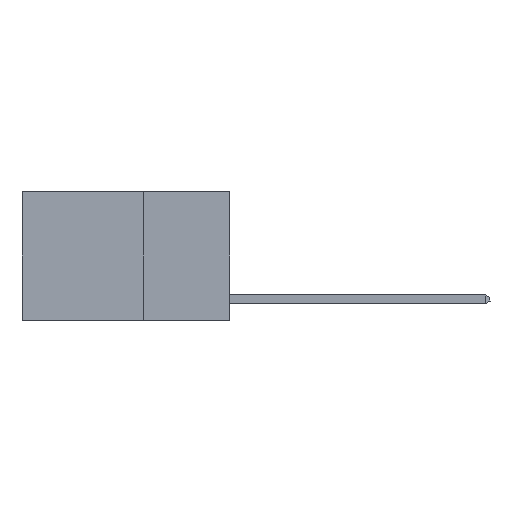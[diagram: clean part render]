
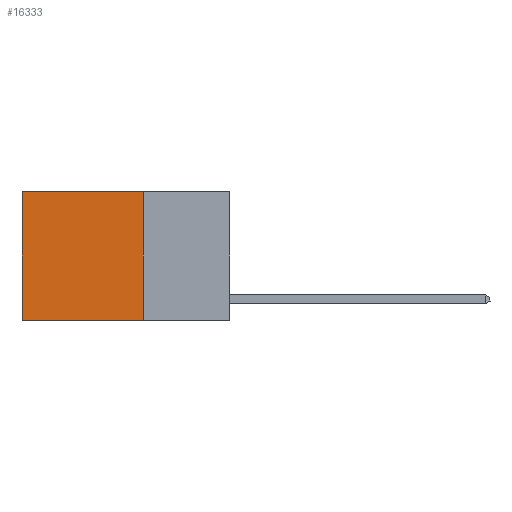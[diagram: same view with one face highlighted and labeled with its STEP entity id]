
A CAD part, left-side view. The second image highlights one B-rep face of the part: STEP entity #16333.
In plain terms, the highlighted planar face has unit normal (-1, 0, 0).
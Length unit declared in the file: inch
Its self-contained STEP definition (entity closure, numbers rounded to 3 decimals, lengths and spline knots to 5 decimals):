
#13 = EDGE_CURVE ( 'NONE', #12201, #6996, #4088, .T. ) ;
#409 = AXIS2_PLACEMENT_3D ( 'NONE', #1195, #7723, #7831 ) ;
#602 = VECTOR ( 'NONE', #15151, 39.37008 ) ;
#702 = CARTESIAN_POINT ( 'NONE',  ( 0.2625, 0.25, 0. ) ) ;
#754 = CARTESIAN_POINT ( 'NONE',  ( 0.2625, 0.25, -0.37 ) ) ;
#1195 = CARTESIAN_POINT ( 'NONE',  ( 0.2625, 0.25, 0. ) ) ;
#2214 = EDGE_CURVE ( 'NONE', #6996, #4383, #11823, .T. ) ;
#2834 = EDGE_LOOP ( 'NONE', ( #11402, #3518, #6866, #16773 ) ) ;
#2910 = CARTESIAN_POINT ( 'NONE',  ( 0.2625, 0.25, -0.37 ) ) ;
#3330 = DIRECTION ( 'NONE',  ( 0., 0., -1. ) ) ;
#3517 = CARTESIAN_POINT ( 'NONE',  ( 0.2625, 0.6, -0.37 ) ) ;
#3518 = ORIENTED_EDGE ( 'NONE', *, *, #5347, .F. ) ;
#3782 = PLANE ( 'NONE',  #409 ) ;
#4088 = LINE ( 'NONE', #12407, #602 ) ;
#4383 = VERTEX_POINT ( 'NONE', #3517 ) ;
#5347 = EDGE_CURVE ( 'NONE', #8418, #4383, #5394, .T. ) ;
#5394 = LINE ( 'NONE', #2910, #11087 ) ;
#6315 = VECTOR ( 'NONE', #3330, 39.37008 ) ;
#6866 = ORIENTED_EDGE ( 'NONE', *, *, #8232, .F. ) ;
#6996 = VERTEX_POINT ( 'NONE', #9057 ) ;
#7723 = DIRECTION ( 'NONE',  ( 1., 0., 0. ) ) ;
#7831 = DIRECTION ( 'NONE',  ( 0., 0., -1. ) ) ;
#8218 = DIRECTION ( 'NONE',  ( 0., 1., 0. ) ) ;
#8232 = EDGE_CURVE ( 'NONE', #12201, #8418, #10728, .T. ) ;
#8418 = VERTEX_POINT ( 'NONE', #754 ) ;
#8505 = CARTESIAN_POINT ( 'NONE',  ( 0.2625, 0.6, 0. ) ) ;
#9057 = CARTESIAN_POINT ( 'NONE',  ( 0.2625, 0.6, 0. ) ) ;
#10728 = LINE ( 'NONE', #702, #11351 ) ;
#11087 = VECTOR ( 'NONE', #8218, 39.37008 ) ;
#11351 = VECTOR ( 'NONE', #12298, 39.37008 ) ;
#11402 = ORIENTED_EDGE ( 'NONE', *, *, #2214, .T. ) ;
#11823 = LINE ( 'NONE', #8505, #6315 ) ;
#12201 = VERTEX_POINT ( 'NONE', #14471 ) ;
#12298 = DIRECTION ( 'NONE',  ( 0., 0., -1. ) ) ;
#12407 = CARTESIAN_POINT ( 'NONE',  ( 0.2625, 0.25, 0. ) ) ;
#13251 = FACE_OUTER_BOUND ( 'NONE', #2834, .T. ) ;
#14471 = CARTESIAN_POINT ( 'NONE',  ( 0.2625, 0.25, 0. ) ) ;
#15151 = DIRECTION ( 'NONE',  ( 0., 1., 0. ) ) ;
#16333 = ADVANCED_FACE ( 'NONE', ( #13251 ), #3782, .F. ) ;
#16773 = ORIENTED_EDGE ( 'NONE', *, *, #13, .T. ) ;
